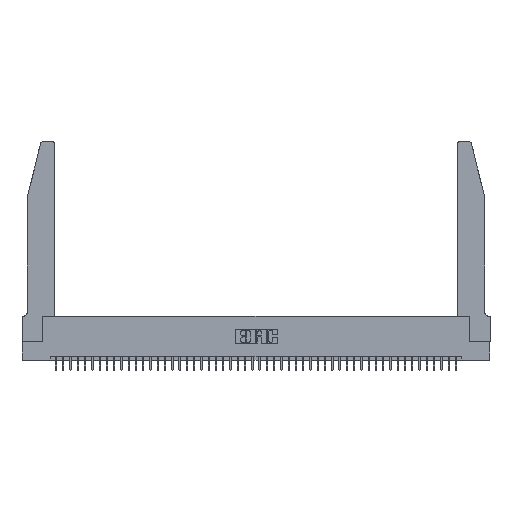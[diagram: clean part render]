
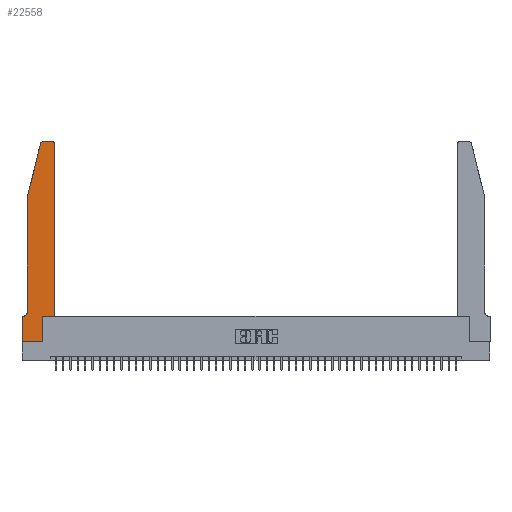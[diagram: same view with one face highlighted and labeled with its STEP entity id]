
A CAD part, top view. The second image highlights one B-rep face of the part: STEP entity #22558.
In plain terms, the highlighted planar face has unit normal (0, 0, 1).
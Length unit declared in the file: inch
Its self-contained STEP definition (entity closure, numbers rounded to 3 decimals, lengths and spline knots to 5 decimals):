
#1259 = CARTESIAN_POINT ( 'NONE',  ( 0.284, 2.75, 0.37 ) ) ;
#1917 = VERTEX_POINT ( 'NONE', #29682 ) ;
#2316 = EDGE_CURVE ( 'NONE', #1917, #30690, #17141, .T. ) ;
#2736 = DIRECTION ( 'NONE',  ( 0., 0., -1. ) ) ;
#2975 = DIRECTION ( 'NONE',  ( 1., 0., 0. ) ) ;
#2978 = CIRCLE ( 'NONE', #29519, 0.07 ) ;
#3108 = LINE ( 'NONE', #21404, #21409 ) ;
#3274 = LINE ( 'NONE', #41050, #6891 ) ;
#3721 = DIRECTION ( 'NONE',  ( 0., 0., 1. ) ) ;
#4593 = VERTEX_POINT ( 'NONE', #40229 ) ;
#4622 = EDGE_CURVE ( 'NONE', #34811, #29999, #15787, .T. ) ;
#4647 = CARTESIAN_POINT ( 'NONE',  ( 0.25487, 2.72718, 0.37 ) ) ;
#4969 = DIRECTION ( 'NONE',  ( 0., 1., 0. ) ) ;
#5221 = EDGE_CURVE ( 'NONE', #19477, #35291, #8972, .T. ) ;
#6891 = VECTOR ( 'NONE', #19403, 39.37008 ) ;
#7195 = FACE_OUTER_BOUND ( 'NONE', #40428, .T. ) ;
#7631 = CARTESIAN_POINT ( 'NONE',  ( 0.0755, 0.42, 0.37 ) ) ;
#8208 = DIRECTION ( 'NONE',  ( 0., -1., 0. ) ) ;
#8950 = DIRECTION ( 'NONE',  ( 1., 0., 0. ) ) ;
#8972 = LINE ( 'NONE', #9440, #37774 ) ;
#9407 = ORIENTED_EDGE ( 'NONE', *, *, #42836, .T. ) ;
#9440 = CARTESIAN_POINT ( 'NONE',  ( 0.2865, 0.35, 0.37 ) ) ;
#9850 = ORIENTED_EDGE ( 'NONE', *, *, #42049, .T. ) ;
#10036 = VERTEX_POINT ( 'NONE', #32521 ) ;
#11456 = EDGE_CURVE ( 'NONE', #29999, #10036, #30598, .T. ) ;
#12048 = LINE ( 'NONE', #19213, #37375 ) ;
#12135 = CARTESIAN_POINT ( 'NONE',  ( 0.284, 2.72, 0.37 ) ) ;
#13054 = ORIENTED_EDGE ( 'NONE', *, *, #11456, .T. ) ;
#13431 = VERTEX_POINT ( 'NONE', #7631 ) ;
#13714 = DIRECTION ( 'NONE',  ( 0., -1., 0. ) ) ;
#13834 = EDGE_CURVE ( 'NONE', #46455, #4593, #15834, .T. ) ;
#14857 = ORIENTED_EDGE ( 'NONE', *, *, #40110, .T. ) ;
#15787 = CIRCLE ( 'NONE', #44648, 0.03 ) ;
#15834 = LINE ( 'NONE', #40346, #44996 ) ;
#16051 = DIRECTION ( 'NONE',  ( 1., 0., 0. ) ) ;
#16727 = CARTESIAN_POINT ( 'NONE',  ( 0.0055, 0.35, 0.37 ) ) ;
#17141 = CIRCLE ( 'NONE', #26267, 0.03 ) ;
#18206 = LINE ( 'NONE', #32472, #29700 ) ;
#18271 = CARTESIAN_POINT ( 'NONE',  ( 0.0755, 0.35, 0.37 ) ) ;
#18498 = LINE ( 'NONE', #18271, #43949 ) ;
#18738 = DIRECTION ( 'NONE',  ( -1., 0., 0. ) ) ;
#18943 = CARTESIAN_POINT ( 'NONE',  ( 0.2865, 0.35, 0.37 ) ) ;
#19059 = ORIENTED_EDGE ( 'NONE', *, *, #43872, .T. ) ;
#19213 = CARTESIAN_POINT ( 'NONE',  ( 0.4505, 0.35, 0.37 ) ) ;
#19403 = DIRECTION ( 'NONE',  ( 0., 1., 0. ) ) ;
#19477 = VERTEX_POINT ( 'NONE', #33376 ) ;
#20152 = CARTESIAN_POINT ( 'NONE',  ( 0.0755, 2., 0.37 ) ) ;
#21404 = CARTESIAN_POINT ( 'NONE',  ( 0., 0., 0.37 ) ) ;
#21409 = VECTOR ( 'NONE', #24985, 39.37008 ) ;
#21498 = PLANE ( 'NONE',  #41229 ) ;
#21557 = EDGE_CURVE ( 'NONE', #4593, #19477, #3108, .T. ) ;
#22400 = DIRECTION ( 'NONE',  ( 0., 0., 1. ) ) ;
#22558 = ADVANCED_FACE ( 'NONE', ( #7195 ), #21498, .T. ) ;
#24888 = ORIENTED_EDGE ( 'NONE', *, *, #5221, .T. ) ;
#24985 = DIRECTION ( 'NONE',  ( 1., 0., 0. ) ) ;
#25409 = ORIENTED_EDGE ( 'NONE', *, *, #2316, .T. ) ;
#25936 = LINE ( 'NONE', #40416, #27312 ) ;
#26267 = AXIS2_PLACEMENT_3D ( 'NONE', #36269, #3721, #16051 ) ;
#26676 = DIRECTION ( 'NONE',  ( 1., 0., 0. ) ) ;
#27059 = DIRECTION ( 'NONE',  ( -0.239, -0.971, 0. ) ) ;
#27312 = VECTOR ( 'NONE', #34457, 39.37008 ) ;
#29519 = AXIS2_PLACEMENT_3D ( 'NONE', #38153, #2736, #38622 ) ;
#29531 = ORIENTED_EDGE ( 'NONE', *, *, #33461, .T. ) ;
#29682 = CARTESIAN_POINT ( 'NONE',  ( 0.4505, 2.72, 0.37 ) ) ;
#29700 = VECTOR ( 'NONE', #13714, 39.37008 ) ;
#29999 = VERTEX_POINT ( 'NONE', #4647 ) ;
#30598 = LINE ( 'NONE', #20152, #37209 ) ;
#30690 = VERTEX_POINT ( 'NONE', #36640 ) ;
#32472 = CARTESIAN_POINT ( 'NONE',  ( 0.0755, 2., 0.37 ) ) ;
#32521 = CARTESIAN_POINT ( 'NONE',  ( 0.0755, 2., 0.37 ) ) ;
#32582 = EDGE_CURVE ( 'NONE', #30690, #34811, #25936, .T. ) ;
#33376 = CARTESIAN_POINT ( 'NONE',  ( 0.2865, 0., 0.37 ) ) ;
#33461 = EDGE_CURVE ( 'NONE', #13431, #37128, #2978, .T. ) ;
#33873 = ORIENTED_EDGE ( 'NONE', *, *, #13834, .T. ) ;
#34457 = DIRECTION ( 'NONE',  ( -1., 0., 0. ) ) ;
#34811 = VERTEX_POINT ( 'NONE', #1259 ) ;
#35291 = VERTEX_POINT ( 'NONE', #18943 ) ;
#36269 = CARTESIAN_POINT ( 'NONE',  ( 0.4205, 2.72, 0.37 ) ) ;
#36345 = CARTESIAN_POINT ( 'NONE',  ( 0.4505, 0.35, 0.37 ) ) ;
#36407 = VERTEX_POINT ( 'NONE', #36345 ) ;
#36640 = CARTESIAN_POINT ( 'NONE',  ( 0.4205, 2.75, 0.37 ) ) ;
#37128 = VERTEX_POINT ( 'NONE', #16727 ) ;
#37209 = VECTOR ( 'NONE', #27059, 39.37008 ) ;
#37375 = VECTOR ( 'NONE', #8950, 39.37008 ) ;
#37774 = VECTOR ( 'NONE', #4969, 39.37008 ) ;
#38153 = CARTESIAN_POINT ( 'NONE',  ( 0.0055, 0.42, 0.37 ) ) ;
#38622 = DIRECTION ( 'NONE',  ( -1., 0., 0. ) ) ;
#39066 = CARTESIAN_POINT ( 'NONE',  ( 0., 0.35, 0.37 ) ) ;
#39336 = CARTESIAN_POINT ( 'NONE',  ( 0., 0.35, 0.37 ) ) ;
#39793 = DIRECTION ( 'NONE',  ( 0., 0., 1. ) ) ;
#40110 = EDGE_CURVE ( 'NONE', #37128, #46455, #18498, .T. ) ;
#40229 = CARTESIAN_POINT ( 'NONE',  ( 0., 0., 0.37 ) ) ;
#40346 = CARTESIAN_POINT ( 'NONE',  ( 0., 0., 0.37 ) ) ;
#40416 = CARTESIAN_POINT ( 'NONE',  ( 0.2605, 2.75, 0.37 ) ) ;
#40428 = EDGE_LOOP ( 'NONE', ( #40910, #44074, #13054, #9407, #29531, #14857, #33873, #41298, #24888, #19059, #9850, #25409 ) ) ;
#40910 = ORIENTED_EDGE ( 'NONE', *, *, #32582, .T. ) ;
#41050 = CARTESIAN_POINT ( 'NONE',  ( 0.4505, 0.35, 0.37 ) ) ;
#41229 = AXIS2_PLACEMENT_3D ( 'NONE', #39336, #39793, #2975 ) ;
#41298 = ORIENTED_EDGE ( 'NONE', *, *, #21557, .T. ) ;
#42049 = EDGE_CURVE ( 'NONE', #36407, #1917, #3274, .T. ) ;
#42836 = EDGE_CURVE ( 'NONE', #10036, #13431, #18206, .T. ) ;
#43872 = EDGE_CURVE ( 'NONE', #35291, #36407, #12048, .T. ) ;
#43949 = VECTOR ( 'NONE', #18738, 39.37008 ) ;
#44074 = ORIENTED_EDGE ( 'NONE', *, *, #4622, .T. ) ;
#44648 = AXIS2_PLACEMENT_3D ( 'NONE', #12135, #22400, #26676 ) ;
#44996 = VECTOR ( 'NONE', #8208, 39.37008 ) ;
#46455 = VERTEX_POINT ( 'NONE', #39066 ) ;
